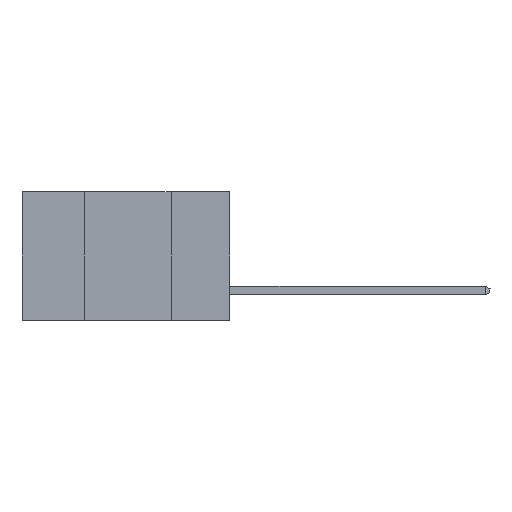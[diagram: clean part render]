
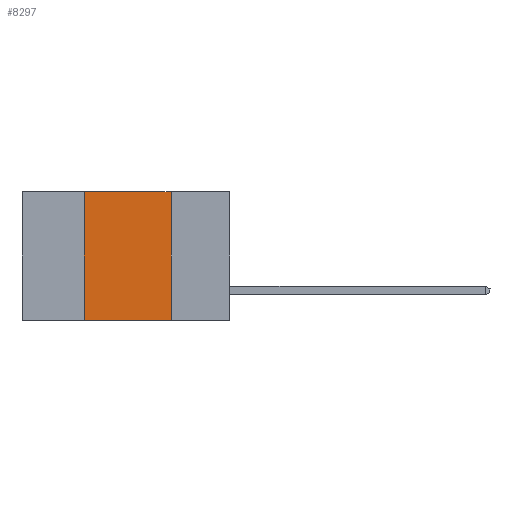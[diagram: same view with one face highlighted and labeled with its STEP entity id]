
A CAD part, left-side view. The second image highlights one B-rep face of the part: STEP entity #8297.
In plain terms, the highlighted planar face has unit normal (-1, 0, 0).
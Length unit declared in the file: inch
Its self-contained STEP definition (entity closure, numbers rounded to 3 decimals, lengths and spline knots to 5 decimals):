
#477 = LINE ( 'NONE', #14351, #7533 ) ;
#497 = ORIENTED_EDGE ( 'NONE', *, *, #2242, .F. ) ;
#633 = CARTESIAN_POINT ( 'NONE',  ( 0., 0.6, 0. ) ) ;
#764 = DIRECTION ( 'NONE',  ( 0., -1., 0. ) ) ;
#1065 = VERTEX_POINT ( 'NONE', #1826 ) ;
#1674 = DIRECTION ( 'NONE',  ( 0., -1., 0. ) ) ;
#1826 = CARTESIAN_POINT ( 'NONE',  ( 0., 0.42, -0.37 ) ) ;
#2231 = ORIENTED_EDGE ( 'NONE', *, *, #12471, .F. ) ;
#2242 = EDGE_CURVE ( 'NONE', #1065, #4901, #5687, .T. ) ;
#2348 = VERTEX_POINT ( 'NONE', #8754 ) ;
#2397 = CARTESIAN_POINT ( 'NONE',  ( 0., 0.42, 0. ) ) ;
#2490 = FACE_OUTER_BOUND ( 'NONE', #11966, .T. ) ;
#2667 = VERTEX_POINT ( 'NONE', #10540 ) ;
#2899 = CARTESIAN_POINT ( 'NONE',  ( 0., 0.17, 0. ) ) ;
#3909 = CARTESIAN_POINT ( 'NONE',  ( 0., 0.6, -0.37 ) ) ;
#3978 = CARTESIAN_POINT ( 'NONE',  ( 0., 0.42, 0. ) ) ;
#4108 = EDGE_CURVE ( 'NONE', #1065, #2667, #14198, .T. ) ;
#4901 = VERTEX_POINT ( 'NONE', #3978 ) ;
#4994 = VECTOR ( 'NONE', #7311, 39.37008 ) ;
#5092 = EDGE_CURVE ( 'NONE', #4901, #2348, #477, .T. ) ;
#5211 = PLANE ( 'NONE',  #14388 ) ;
#5687 = LINE ( 'NONE', #2397, #13193 ) ;
#7311 = DIRECTION ( 'NONE',  ( 0., 0., -1. ) ) ;
#7533 = VECTOR ( 'NONE', #764, 39.37008 ) ;
#8297 = ADVANCED_FACE ( 'NONE', ( #2490 ), #5211, .F. ) ;
#8754 = CARTESIAN_POINT ( 'NONE',  ( 0., 0.17, 0. ) ) ;
#9835 = LINE ( 'NONE', #2899, #4994 ) ;
#9948 = ORIENTED_EDGE ( 'NONE', *, *, #4108, .T. ) ;
#10540 = CARTESIAN_POINT ( 'NONE',  ( 0., 0.17, -0.37 ) ) ;
#10905 = DIRECTION ( 'NONE',  ( 0., 0., 1. ) ) ;
#10967 = ORIENTED_EDGE ( 'NONE', *, *, #5092, .F. ) ;
#11966 = EDGE_LOOP ( 'NONE', ( #2231, #10967, #497, #9948 ) ) ;
#12471 = EDGE_CURVE ( 'NONE', #2348, #2667, #9835, .T. ) ;
#12984 = VECTOR ( 'NONE', #1674, 39.37008 ) ;
#13193 = VECTOR ( 'NONE', #10905, 39.37008 ) ;
#13203 = DIRECTION ( 'NONE',  ( 0., 0., -1. ) ) ;
#14119 = DIRECTION ( 'NONE',  ( 1., 0., 0. ) ) ;
#14198 = LINE ( 'NONE', #3909, #12984 ) ;
#14351 = CARTESIAN_POINT ( 'NONE',  ( 0., 0.6, 0. ) ) ;
#14388 = AXIS2_PLACEMENT_3D ( 'NONE', #633, #14119, #13203 ) ;
